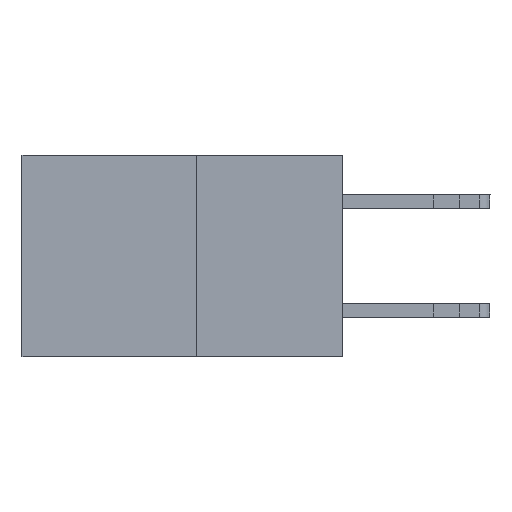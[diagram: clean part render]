
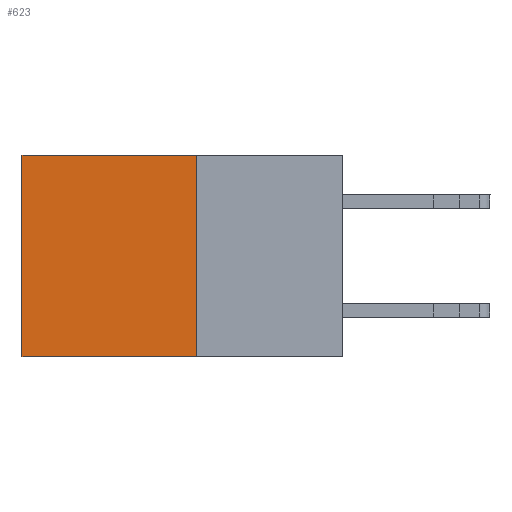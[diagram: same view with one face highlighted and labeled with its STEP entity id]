
A CAD part, left-side view. The second image highlights one B-rep face of the part: STEP entity #623.
In plain terms, the highlighted planar face has unit normal (-1, 0, 0).
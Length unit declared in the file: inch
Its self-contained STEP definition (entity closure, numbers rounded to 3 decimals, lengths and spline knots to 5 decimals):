
#339 = CARTESIAN_POINT ( 'NONE',  ( 0.277, 0.59, -0.37 ) ) ;
#491 = DIRECTION ( 'NONE',  ( 0., 1., 0. ) ) ;
#623 = ADVANCED_FACE ( 'NONE', ( #19666 ), #19836, .F. ) ;
#1142 = EDGE_CURVE ( 'NONE', #22853, #25018, #8485, .T. ) ;
#1147 = CARTESIAN_POINT ( 'NONE',  ( 0.277, 0.27, 0. ) ) ;
#1453 = LINE ( 'NONE', #1147, #21273 ) ;
#2399 = DIRECTION ( 'NONE',  ( 0., 0., -1. ) ) ;
#4921 = EDGE_CURVE ( 'NONE', #22853, #21261, #1453, .T. ) ;
#5050 = LINE ( 'NONE', #339, #22925 ) ;
#6546 = ORIENTED_EDGE ( 'NONE', *, *, #1142, .F. ) ;
#7282 = DIRECTION ( 'NONE',  ( 1., 0., 0. ) ) ;
#8328 = DIRECTION ( 'NONE',  ( 0., 0., -1. ) ) ;
#8485 = LINE ( 'NONE', #26225, #10686 ) ;
#10686 = VECTOR ( 'NONE', #8328, 39.37008 ) ;
#11077 = DIRECTION ( 'NONE',  ( 0., 1., 0. ) ) ;
#11556 = CARTESIAN_POINT ( 'NONE',  ( 0.277, 0.27, -0.37 ) ) ;
#12464 = ORIENTED_EDGE ( 'NONE', *, *, #4921, .T. ) ;
#15259 = CARTESIAN_POINT ( 'NONE',  ( 0.277, 0.27, -0.37 ) ) ;
#16345 = CARTESIAN_POINT ( 'NONE',  ( 0.277, 0.59, 0. ) ) ;
#17284 = DIRECTION ( 'NONE',  ( 0., 0., -1. ) ) ;
#17733 = EDGE_CURVE ( 'NONE', #21261, #30060, #5050, .T. ) ;
#17762 = LINE ( 'NONE', #27671, #30967 ) ;
#18330 = ORIENTED_EDGE ( 'NONE', *, *, #24878, .F. ) ;
#19075 = ORIENTED_EDGE ( 'NONE', *, *, #17733, .T. ) ;
#19666 = FACE_OUTER_BOUND ( 'NONE', #23718, .T. ) ;
#19836 = PLANE ( 'NONE',  #20040 ) ;
#20040 = AXIS2_PLACEMENT_3D ( 'NONE', #15259, #7282, #2399 ) ;
#21261 = VERTEX_POINT ( 'NONE', #16345 ) ;
#21273 = VECTOR ( 'NONE', #11077, 39.37008 ) ;
#22853 = VERTEX_POINT ( 'NONE', #27234 ) ;
#22925 = VECTOR ( 'NONE', #17284, 39.37008 ) ;
#23718 = EDGE_LOOP ( 'NONE', ( #19075, #18330, #6546, #12464 ) ) ;
#24197 = CARTESIAN_POINT ( 'NONE',  ( 0.277, 0.59, -0.37 ) ) ;
#24878 = EDGE_CURVE ( 'NONE', #25018, #30060, #17762, .T. ) ;
#25018 = VERTEX_POINT ( 'NONE', #11556 ) ;
#26225 = CARTESIAN_POINT ( 'NONE',  ( 0.277, 0.27, -0.37 ) ) ;
#27234 = CARTESIAN_POINT ( 'NONE',  ( 0.277, 0.27, 0. ) ) ;
#27671 = CARTESIAN_POINT ( 'NONE',  ( 0.277, 0.27, -0.37 ) ) ;
#30060 = VERTEX_POINT ( 'NONE', #24197 ) ;
#30967 = VECTOR ( 'NONE', #491, 39.37008 ) ;
